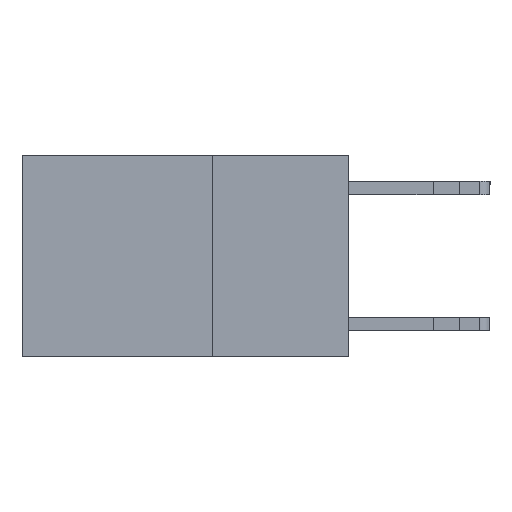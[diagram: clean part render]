
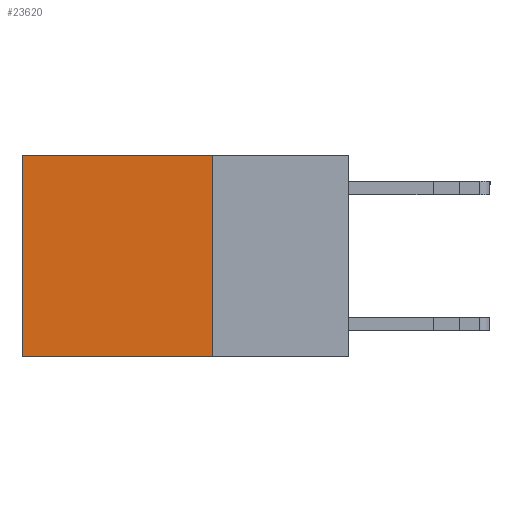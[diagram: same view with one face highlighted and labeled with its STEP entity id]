
A CAD part, left-side view. The second image highlights one B-rep face of the part: STEP entity #23620.
In plain terms, the highlighted planar face has unit normal (-1, 0, 0).
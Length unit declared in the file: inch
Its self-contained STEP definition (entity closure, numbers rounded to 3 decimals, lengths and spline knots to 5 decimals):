
#352 = LINE ( 'NONE', #10728, #966 ) ;
#862 = ORIENTED_EDGE ( 'NONE', *, *, #16194, .T. ) ;
#966 = VECTOR ( 'NONE', #22735, 39.37008 ) ;
#1108 = CARTESIAN_POINT ( 'NONE',  ( 0.2625, 0.25, 0. ) ) ;
#1170 = DIRECTION ( 'NONE',  ( 0., 0., -1. ) ) ;
#1765 = VERTEX_POINT ( 'NONE', #1108 ) ;
#2150 = CARTESIAN_POINT ( 'NONE',  ( 0.2625, 0.25, -0.37 ) ) ;
#2272 = DIRECTION ( 'NONE',  ( 0., 1., 0. ) ) ;
#4893 = VERTEX_POINT ( 'NONE', #15579 ) ;
#5919 = CARTESIAN_POINT ( 'NONE',  ( 0.2625, 0.25, 0. ) ) ;
#6441 = CARTESIAN_POINT ( 'NONE',  ( 0.2625, 0.6, 0. ) ) ;
#7154 = VECTOR ( 'NONE', #2272, 39.37008 ) ;
#7188 = ORIENTED_EDGE ( 'NONE', *, *, #23803, .F. ) ;
#7666 = ORIENTED_EDGE ( 'NONE', *, *, #26162, .F. ) ;
#7884 = FACE_OUTER_BOUND ( 'NONE', #19576, .T. ) ;
#8019 = DIRECTION ( 'NONE',  ( 1., 0., 0. ) ) ;
#9500 = EDGE_CURVE ( 'NONE', #23317, #21394, #23542, .T. ) ;
#10049 = CARTESIAN_POINT ( 'NONE',  ( 0.2625, 0.6, -0.37 ) ) ;
#10116 = AXIS2_PLACEMENT_3D ( 'NONE', #22131, #8019, #13875 ) ;
#10728 = CARTESIAN_POINT ( 'NONE',  ( 0.2625, 0.25, 0. ) ) ;
#11908 = DIRECTION ( 'NONE',  ( 0., 0., -1. ) ) ;
#12882 = VECTOR ( 'NONE', #1170, 39.37008 ) ;
#13875 = DIRECTION ( 'NONE',  ( 0., 0., -1. ) ) ;
#14016 = PLANE ( 'NONE',  #10116 ) ;
#15579 = CARTESIAN_POINT ( 'NONE',  ( 0.2625, 0.25, -0.37 ) ) ;
#16194 = EDGE_CURVE ( 'NONE', #1765, #23317, #352, .T. ) ;
#18528 = LINE ( 'NONE', #2150, #7154 ) ;
#19576 = EDGE_LOOP ( 'NONE', ( #23550, #7188, #7666, #862 ) ) ;
#21276 = VECTOR ( 'NONE', #11908, 39.37008 ) ;
#21394 = VERTEX_POINT ( 'NONE', #10049 ) ;
#22131 = CARTESIAN_POINT ( 'NONE',  ( 0.2625, 0.25, 0. ) ) ;
#22735 = DIRECTION ( 'NONE',  ( 0., 1., 0. ) ) ;
#23317 = VERTEX_POINT ( 'NONE', #6441 ) ;
#23542 = LINE ( 'NONE', #23808, #12882 ) ;
#23550 = ORIENTED_EDGE ( 'NONE', *, *, #9500, .T. ) ;
#23620 = ADVANCED_FACE ( 'NONE', ( #7884 ), #14016, .F. ) ;
#23803 = EDGE_CURVE ( 'NONE', #4893, #21394, #18528, .T. ) ;
#23808 = CARTESIAN_POINT ( 'NONE',  ( 0.2625, 0.6, 0. ) ) ;
#24426 = LINE ( 'NONE', #5919, #21276 ) ;
#26162 = EDGE_CURVE ( 'NONE', #1765, #4893, #24426, .T. ) ;
